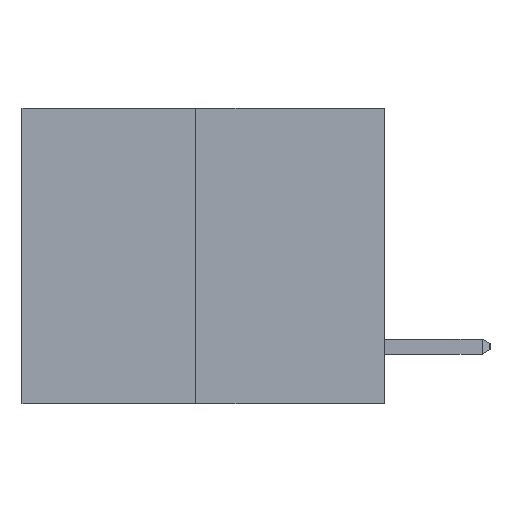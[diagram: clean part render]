
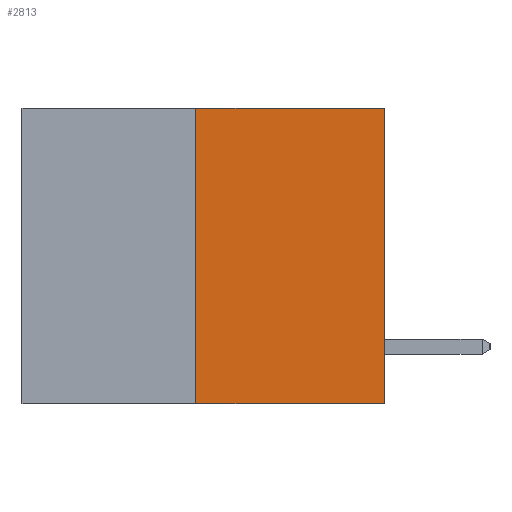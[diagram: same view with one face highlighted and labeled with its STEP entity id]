
A CAD part, left-side view. The second image highlights one B-rep face of the part: STEP entity #2813.
In plain terms, the highlighted planar face has unit normal (-1, 0, 0).
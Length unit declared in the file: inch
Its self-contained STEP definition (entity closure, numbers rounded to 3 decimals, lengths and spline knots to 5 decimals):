
#208 = FACE_OUTER_BOUND ( 'NONE', #2537, .T. ) ;
#531 = VECTOR ( 'NONE', #9918, 39.37008 ) ;
#1478 = CARTESIAN_POINT ( 'NONE',  ( 0., 0., -0.49 ) ) ;
#1606 = ORIENTED_EDGE ( 'NONE', *, *, #18252, .T. ) ;
#2537 = EDGE_LOOP ( 'NONE', ( #12305, #14413, #1606, #14326 ) ) ;
#2813 = ADVANCED_FACE ( 'NONE', ( #208 ), #15800, .F. ) ;
#3216 = DIRECTION ( 'NONE',  ( 0., -1., 0. ) ) ;
#3264 = LINE ( 'NONE', #16058, #12792 ) ;
#3472 = VECTOR ( 'NONE', #5473, 39.37008 ) ;
#3762 = CARTESIAN_POINT ( 'NONE',  ( 0., 0.312, 0. ) ) ;
#3856 = CARTESIAN_POINT ( 'NONE',  ( 0., 0.6, -0.49 ) ) ;
#5473 = DIRECTION ( 'NONE',  ( 0., -1., 0. ) ) ;
#5582 = DIRECTION ( 'NONE',  ( 0., 0., 1. ) ) ;
#5884 = VERTEX_POINT ( 'NONE', #11628 ) ;
#6107 = EDGE_CURVE ( 'NONE', #12871, #10133, #18584, .T. ) ;
#7287 = AXIS2_PLACEMENT_3D ( 'NONE', #15743, #15866, #8347 ) ;
#8347 = DIRECTION ( 'NONE',  ( 0., 0., -1. ) ) ;
#8711 = EDGE_CURVE ( 'NONE', #12871, #16581, #16467, .T. ) ;
#9918 = DIRECTION ( 'NONE',  ( 0., 0., 1. ) ) ;
#10133 = VERTEX_POINT ( 'NONE', #3762 ) ;
#11023 = VECTOR ( 'NONE', #3216, 39.37008 ) ;
#11628 = CARTESIAN_POINT ( 'NONE',  ( 0., 0., 0. ) ) ;
#12231 = EDGE_CURVE ( 'NONE', #10133, #5884, #15910, .T. ) ;
#12305 = ORIENTED_EDGE ( 'NONE', *, *, #6107, .F. ) ;
#12792 = VECTOR ( 'NONE', #5582, 39.37008 ) ;
#12871 = VERTEX_POINT ( 'NONE', #13430 ) ;
#13430 = CARTESIAN_POINT ( 'NONE',  ( 0., 0.312, -0.49 ) ) ;
#14326 = ORIENTED_EDGE ( 'NONE', *, *, #12231, .F. ) ;
#14413 = ORIENTED_EDGE ( 'NONE', *, *, #8711, .T. ) ;
#15743 = CARTESIAN_POINT ( 'NONE',  ( 0., 0.6, 0. ) ) ;
#15800 = PLANE ( 'NONE',  #7287 ) ;
#15866 = DIRECTION ( 'NONE',  ( 1., 0., 0. ) ) ;
#15910 = LINE ( 'NONE', #17821, #11023 ) ;
#16058 = CARTESIAN_POINT ( 'NONE',  ( 0., 0., 0. ) ) ;
#16467 = LINE ( 'NONE', #3856, #3472 ) ;
#16581 = VERTEX_POINT ( 'NONE', #1478 ) ;
#17821 = CARTESIAN_POINT ( 'NONE',  ( 0., 0.6, 0. ) ) ;
#18252 = EDGE_CURVE ( 'NONE', #16581, #5884, #3264, .T. ) ;
#18584 = LINE ( 'NONE', #19061, #531 ) ;
#19061 = CARTESIAN_POINT ( 'NONE',  ( 0., 0.312, -0.49 ) ) ;
